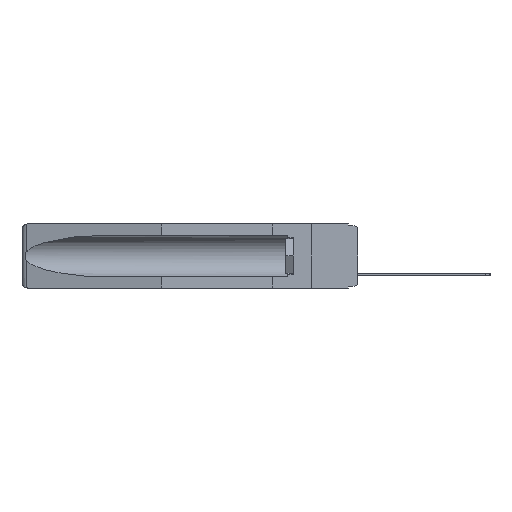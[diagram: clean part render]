
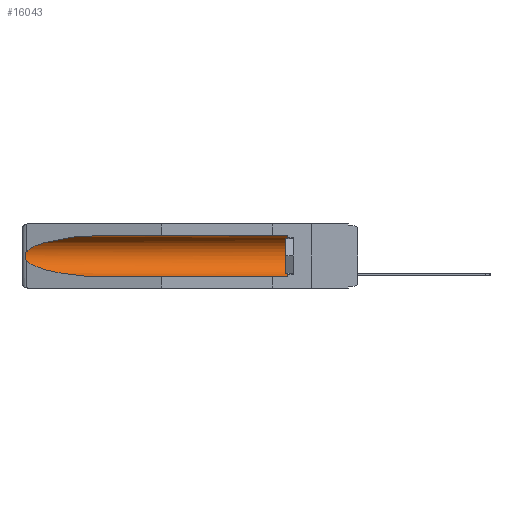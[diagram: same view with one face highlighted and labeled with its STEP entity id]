
A CAD part, left-side view. The second image highlights one B-rep face of the part: STEP entity #16043.
In plain terms, the highlighted cylindrical face has radius 2.857 mm (diameter 5.715 mm), a partial arc.
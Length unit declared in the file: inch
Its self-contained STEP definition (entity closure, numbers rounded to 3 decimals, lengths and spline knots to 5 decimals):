
#628 = CARTESIAN_POINT ( 'NONE',  ( 0.155, -0.30754, -0.059 ) ) ;
#853 = CARTESIAN_POINT ( 'NONE',  ( 0.2673, 1.5327, -0.16383 ) ) ;
#870 = ORIENTED_EDGE ( 'NONE', *, *, #4970, .F. ) ;
#1130 = DIRECTION ( 'NONE',  ( 0., 1., 0. ) ) ;
#1444 = ORIENTED_EDGE ( 'NONE', *, *, #3703, .T. ) ;
#1456 = AXIS2_PLACEMENT_3D ( 'NONE', #11272, #1130, #6952 ) ;
#1474 = CARTESIAN_POINT ( 'NONE',  ( 0.26537, 1.52718, -0.19328 ) ) ;
#2355 = CARTESIAN_POINT ( 'NONE',  ( 0.2675, 1.53308, -0.17534 ) ) ;
#2739 = ORIENTED_EDGE ( 'NONE', *, *, #5417, .T. ) ;
#2849 = DIRECTION ( 'NONE',  ( 0., -1., 0. ) ) ;
#3120 = CYLINDRICAL_SURFACE ( 'NONE', #1456, 0.1125 ) ;
#3476 = VERTEX_POINT ( 'NONE', #8123 ) ;
#3702 = CARTESIAN_POINT ( 'NONE',  ( 0.26597, 1.52961, -0.15275 ) ) ;
#3703 = EDGE_CURVE ( 'NONE', #15813, #3476, #5534, .T. ) ;
#3832 = CARTESIAN_POINT ( 'NONE',  ( 0.26655, 1.53094, -0.18657 ) ) ;
#4323 = CARTESIAN_POINT ( 'NONE',  ( 0.26537, 1.52718, -0.14972 ) ) ;
#4892 = B_SPLINE_CURVE_WITH_KNOTS ( 'NONE', 3,
 ( #6687, #3702, #9552, #853, #11016, #2355, #12399, #3832, #13775, #5283 ),
 .UNSPECIFIED., .F., .F.,
 ( 4, 2, 2, 2, 4 ),
 ( 0., 0.00029, 0.00058, 0.00087, 0.00117 ),
 .UNSPECIFIED. ) ;
#4970 = EDGE_CURVE ( 'NONE', #10412, #12118, #13927, .T. ) ;
#5108 = EDGE_LOOP ( 'NONE', ( #1444, #6273, #12273, #870, #2739, #6392 ) ) ;
#5283 = CARTESIAN_POINT ( 'NONE',  ( 0.26537, 1.52718, -0.19328 ) ) ;
#5417 = EDGE_CURVE ( 'NONE', #10412, #5579, #7306, .T. ) ;
#5534 =( BOUNDED_CURVE ( )  B_SPLINE_CURVE ( 3, ( #18135, #17390, #17470, #4323 ),
 .UNSPECIFIED., .F., .F. ) 
 B_SPLINE_CURVE_WITH_KNOTS ( ( 4, 4 ),
 ( 4.71239, 6.08839 ),
 .UNSPECIFIED. ) 
 CURVE ( )  GEOMETRIC_REPRESENTATION_ITEM ( )  RATIONAL_B_SPLINE_CURVE ( ( 1., 0.848, 0.848, 1. ) ) 
 REPRESENTATION_ITEM ( '' )  );
#5579 = VERTEX_POINT ( 'NONE', #14524 ) ;
#6273 = ORIENTED_EDGE ( 'NONE', *, *, #12495, .T. ) ;
#6392 = ORIENTED_EDGE ( 'NONE', *, *, #15298, .T. ) ;
#6687 = CARTESIAN_POINT ( 'NONE',  ( 0.26537, 1.52718, -0.14972 ) ) ;
#6738 = VECTOR ( 'NONE', #13574, 39.37008 ) ;
#6952 = DIRECTION ( 'NONE',  ( 0., 0., 1. ) ) ;
#7246 = CARTESIAN_POINT ( 'NONE',  ( 0.155, 1.07973, -0.284 ) ) ;
#7306 = CIRCLE ( 'NONE', #13114, 0.1125 ) ;
#8123 = CARTESIAN_POINT ( 'NONE',  ( 0.26537, 1.52718, -0.14972 ) ) ;
#9266 =( BOUNDED_CURVE ( )  B_SPLINE_CURVE ( 3, ( #16883, #14235, #15591, #7246 ),
 .UNSPECIFIED., .F., .F. ) 
 B_SPLINE_CURVE_WITH_KNOTS ( ( 4, 4 ),
 ( 0.1948, 1.5708 ),
 .UNSPECIFIED. ) 
 CURVE ( )  GEOMETRIC_REPRESENTATION_ITEM ( )  RATIONAL_B_SPLINE_CURVE ( ( 1., 0.848, 0.848, 1. ) ) 
 REPRESENTATION_ITEM ( '' )  );
#9287 = CARTESIAN_POINT ( 'NONE',  ( 0.155, 1.07973, -0.059 ) ) ;
#9552 = CARTESIAN_POINT ( 'NONE',  ( 0.26654, 1.53092, -0.15636 ) ) ;
#10223 = VECTOR ( 'NONE', #13196, 39.37008 ) ;
#10376 = CARTESIAN_POINT ( 'NONE',  ( 0.155, -0.30754, -0.284 ) ) ;
#10412 = VERTEX_POINT ( 'NONE', #15714 ) ;
#10528 = LINE ( 'NONE', #628, #6738 ) ;
#11016 = CARTESIAN_POINT ( 'NONE',  ( 0.2675, 1.53308, -0.16763 ) ) ;
#11272 = CARTESIAN_POINT ( 'NONE',  ( 0.155, -0.30754, -0.1715 ) ) ;
#11499 = CARTESIAN_POINT ( 'NONE',  ( 0.155, 0.126, -0.1715 ) ) ;
#12118 = VERTEX_POINT ( 'NONE', #16889 ) ;
#12273 = ORIENTED_EDGE ( 'NONE', *, *, #12799, .T. ) ;
#12399 = CARTESIAN_POINT ( 'NONE',  ( 0.2673, 1.53269, -0.17917 ) ) ;
#12495 = EDGE_CURVE ( 'NONE', #3476, #17190, #4892, .T. ) ;
#12799 = EDGE_CURVE ( 'NONE', #17190, #12118, #9266, .T. ) ;
#12869 = DIRECTION ( 'NONE',  ( 0., 0., 1. ) ) ;
#13114 = AXIS2_PLACEMENT_3D ( 'NONE', #11499, #2849, #12869 ) ;
#13196 = DIRECTION ( 'NONE',  ( 0., 1., 0. ) ) ;
#13574 = DIRECTION ( 'NONE',  ( 0., 1., 0. ) ) ;
#13775 = CARTESIAN_POINT ( 'NONE',  ( 0.26597, 1.5296, -0.19026 ) ) ;
#13927 = LINE ( 'NONE', #10376, #10223 ) ;
#14235 = CARTESIAN_POINT ( 'NONE',  ( 0.25451, 1.48313, -0.24835 ) ) ;
#14444 = FACE_OUTER_BOUND ( 'NONE', #5108, .T. ) ;
#14524 = CARTESIAN_POINT ( 'NONE',  ( 0.155, 0.126, -0.059 ) ) ;
#15298 = EDGE_CURVE ( 'NONE', #5579, #15813, #10528, .T. ) ;
#15591 = CARTESIAN_POINT ( 'NONE',  ( 0.21114, 1.30732, -0.284 ) ) ;
#15714 = CARTESIAN_POINT ( 'NONE',  ( 0.155, 0.126, -0.284 ) ) ;
#15813 = VERTEX_POINT ( 'NONE', #9287 ) ;
#16043 = ADVANCED_FACE ( 'NONE', ( #14444 ), #3120, .F. ) ;
#16883 = CARTESIAN_POINT ( 'NONE',  ( 0.26537, 1.52718, -0.19328 ) ) ;
#16889 = CARTESIAN_POINT ( 'NONE',  ( 0.155, 1.07973, -0.284 ) ) ;
#17190 = VERTEX_POINT ( 'NONE', #1474 ) ;
#17390 = CARTESIAN_POINT ( 'NONE',  ( 0.21114, 1.30732, -0.059 ) ) ;
#17470 = CARTESIAN_POINT ( 'NONE',  ( 0.25451, 1.48313, -0.09465 ) ) ;
#18135 = CARTESIAN_POINT ( 'NONE',  ( 0.155, 1.07973, -0.059 ) ) ;
